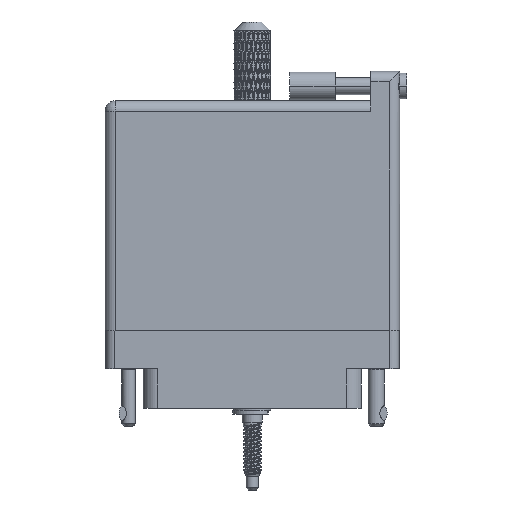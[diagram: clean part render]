
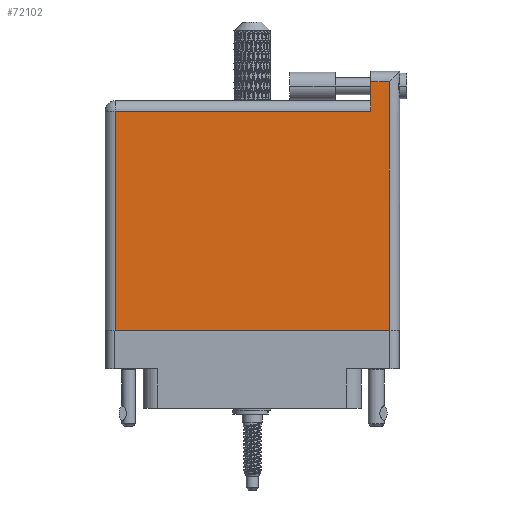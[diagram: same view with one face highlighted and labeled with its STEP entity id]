
A CAD part, front view. The second image highlights one B-rep face of the part: STEP entity #72102.
In plain terms, the highlighted face is planar.
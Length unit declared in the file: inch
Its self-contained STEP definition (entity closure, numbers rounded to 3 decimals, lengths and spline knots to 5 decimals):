
#378 = LINE ( 'NONE', #87613, #111696 ) ;
#2564 = VECTOR ( 'NONE', #46707, 39.37008 ) ;
#4306 = VECTOR ( 'NONE', #110212, 39.37008 ) ;
#8852 = LINE ( 'NONE', #63940, #107697 ) ;
#13697 = VECTOR ( 'NONE', #43450, 39.37008 ) ;
#13884 = LINE ( 'NONE', #39480, #4306 ) ;
#14338 = VERTEX_POINT ( 'NONE', #27725 ) ;
#27725 = CARTESIAN_POINT ( 'NONE',  ( 1.811, 1.696, 0. ) ) ;
#29048 = ORIENTED_EDGE ( 'NONE', *, *, #58889, .T. ) ;
#31652 = ORIENTED_EDGE ( 'NONE', *, *, #49042, .T. ) ;
#31844 = FACE_OUTER_BOUND ( 'NONE', #34534, .T. ) ;
#32530 = VERTEX_POINT ( 'NONE', #109198 ) ;
#34249 = CARTESIAN_POINT ( 'NONE',  ( 0.07, 0., 0. ) ) ;
#34534 = EDGE_LOOP ( 'NONE', ( #41783, #89519, #40641, #95329, #29048, #31652 ) ) ;
#39480 = CARTESIAN_POINT ( 'NONE',  ( 0., 1.696, 0. ) ) ;
#40641 = ORIENTED_EDGE ( 'NONE', *, *, #93386, .T. ) ;
#41269 = VERTEX_POINT ( 'NONE', #61023 ) ;
#41783 = ORIENTED_EDGE ( 'NONE', *, *, #113393, .T. ) ;
#43450 = DIRECTION ( 'NONE',  ( 0., -1., 0. ) ) ;
#43454 = LINE ( 'NONE', #104973, #61265 ) ;
#46707 = DIRECTION ( 'NONE',  ( 0., -1., 0. ) ) ;
#49042 = EDGE_CURVE ( 'NONE', #78976, #50059, #67112, .T. ) ;
#50059 = VERTEX_POINT ( 'NONE', #83827 ) ;
#51958 = DIRECTION ( 'NONE',  ( 0., 1., 0. ) ) ;
#54832 = DIRECTION ( 'NONE',  ( -1., 0., 0. ) ) ;
#55205 = DIRECTION ( 'NONE',  ( 0., 0., -1. ) ) ;
#58889 = EDGE_CURVE ( 'NONE', #65860, #78976, #8852, .T. ) ;
#61023 = CARTESIAN_POINT ( 'NONE',  ( 1.938, 1.696, 0. ) ) ;
#61265 = VECTOR ( 'NONE', #51958, 39.37008 ) ;
#61364 = EDGE_CURVE ( 'NONE', #32530, #41269, #43454, .T. ) ;
#61735 = CARTESIAN_POINT ( 'NONE',  ( 0.07, 1.496, 0. ) ) ;
#63940 = CARTESIAN_POINT ( 'NONE',  ( 0., 1.496, 0. ) ) ;
#65860 = VERTEX_POINT ( 'NONE', #98886 ) ;
#66903 = EDGE_CURVE ( 'NONE', #14338, #65860, #107042, .T. ) ;
#67112 = LINE ( 'NONE', #34249, #13697 ) ;
#71028 = DIRECTION ( 'NONE',  ( 1., 0., 0. ) ) ;
#72003 = DIRECTION ( 'NONE',  ( -1., 0., 0. ) ) ;
#72102 = ADVANCED_FACE ( 'NONE', ( #31844 ), #90095, .F. ) ;
#78976 = VERTEX_POINT ( 'NONE', #61735 ) ;
#81897 = CARTESIAN_POINT ( 'NONE',  ( 1.811, 1.766, 0. ) ) ;
#83827 = CARTESIAN_POINT ( 'NONE',  ( 0.07, 0., 0. ) ) ;
#87613 = CARTESIAN_POINT ( 'NONE',  ( 0., 0., 0. ) ) ;
#88960 = CARTESIAN_POINT ( 'NONE',  ( 0., 1.566, 0. ) ) ;
#89519 = ORIENTED_EDGE ( 'NONE', *, *, #61364, .T. ) ;
#90095 = PLANE ( 'NONE',  #91504 ) ;
#91504 = AXIS2_PLACEMENT_3D ( 'NONE', #88960, #55205, #54832 ) ;
#93386 = EDGE_CURVE ( 'NONE', #41269, #14338, #13884, .T. ) ;
#95329 = ORIENTED_EDGE ( 'NONE', *, *, #66903, .T. ) ;
#98886 = CARTESIAN_POINT ( 'NONE',  ( 1.811, 1.496, 0. ) ) ;
#104973 = CARTESIAN_POINT ( 'NONE',  ( 1.938, 1.766, 0. ) ) ;
#107042 = LINE ( 'NONE', #81897, #2564 ) ;
#107697 = VECTOR ( 'NONE', #72003, 39.37008 ) ;
#109198 = CARTESIAN_POINT ( 'NONE',  ( 1.938, 0., 0. ) ) ;
#110212 = DIRECTION ( 'NONE',  ( -1., 0., 0. ) ) ;
#111696 = VECTOR ( 'NONE', #71028, 39.37008 ) ;
#113393 = EDGE_CURVE ( 'NONE', #50059, #32530, #378, .T. ) ;
